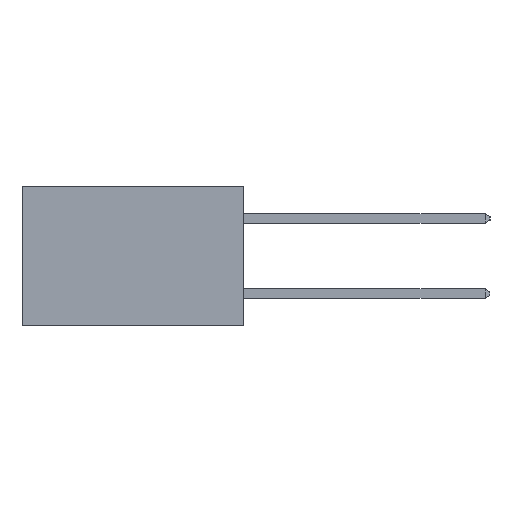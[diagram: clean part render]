
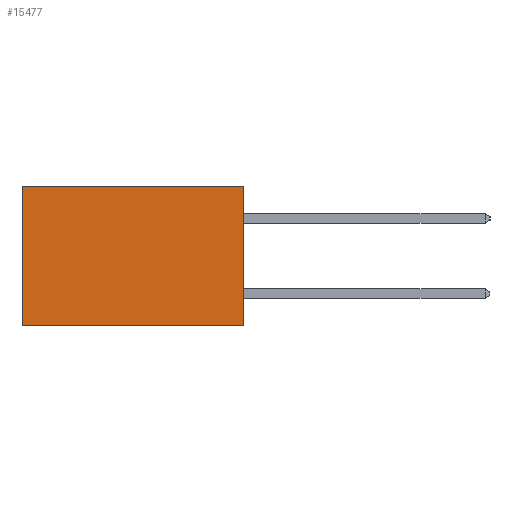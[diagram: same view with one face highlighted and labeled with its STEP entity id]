
A CAD part, left-side view. The second image highlights one B-rep face of the part: STEP entity #15477.
In plain terms, the highlighted planar face has unit normal (-1, 0, 0).
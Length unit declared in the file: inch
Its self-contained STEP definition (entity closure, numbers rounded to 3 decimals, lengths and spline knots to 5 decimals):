
#101 = EDGE_LOOP ( 'NONE', ( #1685, #10007, #3667, #830 ) ) ;
#620 = DIRECTION ( 'NONE',  ( 0., 1., 0. ) ) ;
#830 = ORIENTED_EDGE ( 'NONE', *, *, #15853, .T. ) ;
#930 = CARTESIAN_POINT ( 'NONE',  ( 0.277, 0., -0.37 ) ) ;
#1439 = LINE ( 'NONE', #930, #4685 ) ;
#1575 = DIRECTION ( 'NONE',  ( 0., 0., -1. ) ) ;
#1685 = ORIENTED_EDGE ( 'NONE', *, *, #8527, .T. ) ;
#2221 = EDGE_CURVE ( 'NONE', #16575, #6903, #1439, .T. ) ;
#3595 = CARTESIAN_POINT ( 'NONE',  ( 0.277, 0., -0.37 ) ) ;
#3667 = ORIENTED_EDGE ( 'NONE', *, *, #4155, .F. ) ;
#4155 = EDGE_CURVE ( 'NONE', #11844, #16575, #16910, .T. ) ;
#4621 = FACE_OUTER_BOUND ( 'NONE', #101, .T. ) ;
#4685 = VECTOR ( 'NONE', #620, 39.37008 ) ;
#4968 = DIRECTION ( 'NONE',  ( 1., 0., 0. ) ) ;
#4971 = DIRECTION ( 'NONE',  ( 0., 0., -1. ) ) ;
#4993 = CARTESIAN_POINT ( 'NONE',  ( 0.277, 0., -0.37 ) ) ;
#5710 = LINE ( 'NONE', #9750, #13255 ) ;
#6169 = CARTESIAN_POINT ( 'NONE',  ( 0.277, 0.59, 0. ) ) ;
#6893 = AXIS2_PLACEMENT_3D ( 'NONE', #3595, #4968, #14301 ) ;
#6903 = VERTEX_POINT ( 'NONE', #7798 ) ;
#7798 = CARTESIAN_POINT ( 'NONE',  ( 0.277, 0.59, -0.37 ) ) ;
#8344 = DIRECTION ( 'NONE',  ( 0., 1., 0. ) ) ;
#8527 = EDGE_CURVE ( 'NONE', #11263, #6903, #5710, .T. ) ;
#9633 = CARTESIAN_POINT ( 'NONE',  ( 0.277, 0., 0. ) ) ;
#9750 = CARTESIAN_POINT ( 'NONE',  ( 0.277, 0.59, -0.37 ) ) ;
#9895 = VECTOR ( 'NONE', #4971, 39.37008 ) ;
#9898 = LINE ( 'NONE', #9633, #13415 ) ;
#10007 = ORIENTED_EDGE ( 'NONE', *, *, #2221, .F. ) ;
#11263 = VERTEX_POINT ( 'NONE', #6169 ) ;
#11646 = PLANE ( 'NONE',  #6893 ) ;
#11844 = VERTEX_POINT ( 'NONE', #15292 ) ;
#13255 = VECTOR ( 'NONE', #1575, 39.37008 ) ;
#13415 = VECTOR ( 'NONE', #8344, 39.37008 ) ;
#13802 = CARTESIAN_POINT ( 'NONE',  ( 0.277, 0., -0.37 ) ) ;
#14301 = DIRECTION ( 'NONE',  ( 0., 0., -1. ) ) ;
#15292 = CARTESIAN_POINT ( 'NONE',  ( 0.277, 0., 0. ) ) ;
#15477 = ADVANCED_FACE ( 'NONE', ( #4621 ), #11646, .F. ) ;
#15853 = EDGE_CURVE ( 'NONE', #11844, #11263, #9898, .T. ) ;
#16575 = VERTEX_POINT ( 'NONE', #13802 ) ;
#16910 = LINE ( 'NONE', #4993, #9895 ) ;
